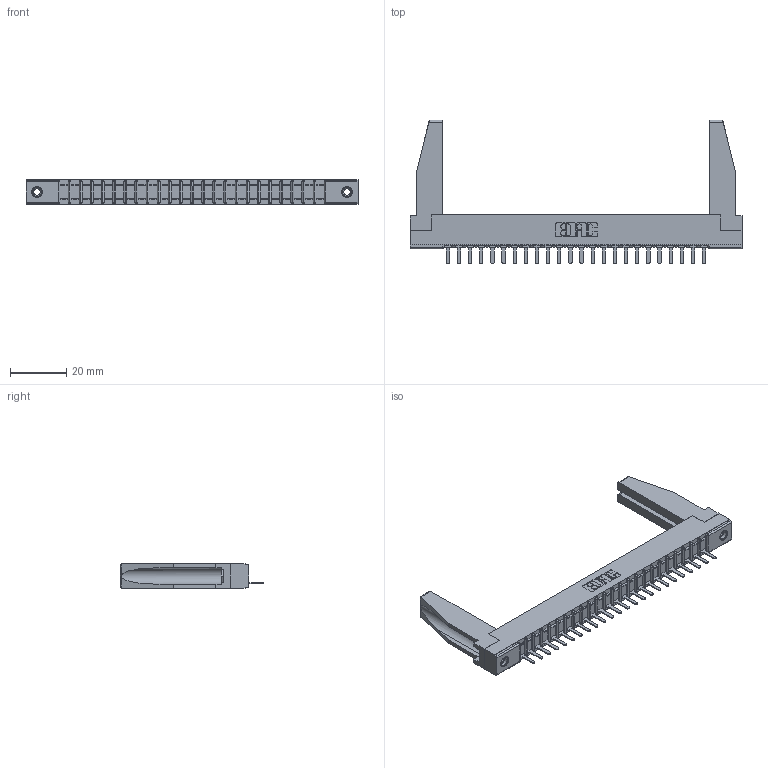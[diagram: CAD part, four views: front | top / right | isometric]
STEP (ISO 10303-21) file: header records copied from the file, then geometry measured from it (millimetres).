
FILE_DESCRIPTION (( 'STEP AP203' ), '1' );
FILE_NAME ('307-024-421-178.STEP', '2020-09-27T11:24:13', ( '' ), ( '' ), 'SwSTEP 2.0', 'SolidWorks 2020', '' );
FILE_SCHEMA (( 'CONFIG_CONTROL_DESIGN' ));
Length unit declared in the file: inch
Products named in the file (5): 307-024-421-178; 307-220-078; 345-250-001_345-250-001-102; 307 Part_.156 Dia Mounting Holes; 307-290-002_521
Assembly tree (29 placements, depth 2):
  307-024-421-178
    307 Part_.156 Dia Mounting Holes
    307-290-002_521  x24
    307-220-078  x2
    345-250-001_345-250-001-102  x2
Bounding box: 118.11 x 51.13 x 8.71 mm (x, y, z)
Volume: 11793.2 mm3; surface area: 18133 mm2
Topology: 29 solids, 29 shells, 2049 faces, 6221 edges, 4070 vertices
Faces by surface type: plane 1234, cylinder 749, sphere 50, cone 12, torus 4
Entity records: 25951 total; most frequent: CARTESIAN_POINT 4374, ORIENTED_EDGE 4320, DIRECTION 4214, EDGE_CURVE 2160, VECTOR 1650, LINE 1650, VERTEX_POINT 1400, AXIS2_PLACEMENT_3D 1282
